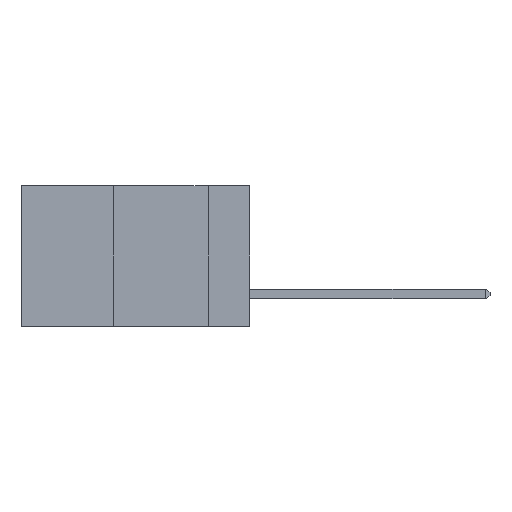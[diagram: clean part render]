
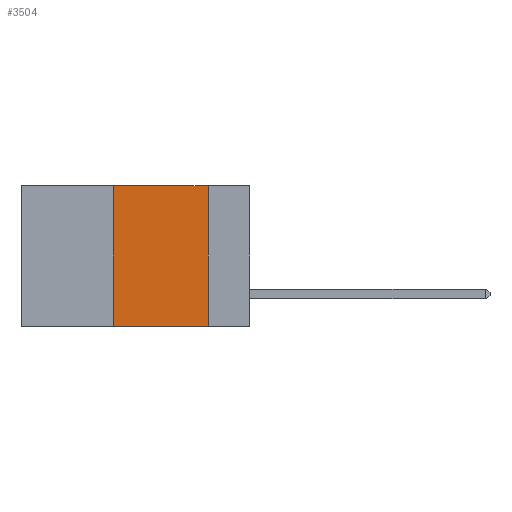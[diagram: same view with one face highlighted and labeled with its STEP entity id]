
A CAD part, left-side view. The second image highlights one B-rep face of the part: STEP entity #3504.
In plain terms, the highlighted planar face has unit normal (-1, 0, 0).
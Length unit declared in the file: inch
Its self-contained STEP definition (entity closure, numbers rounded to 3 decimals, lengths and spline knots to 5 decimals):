
#342 = CARTESIAN_POINT ( 'NONE',  ( 0., 0.36, 0. ) ) ;
#497 = CARTESIAN_POINT ( 'NONE',  ( 0., 0.36, 0. ) ) ;
#803 = VECTOR ( 'NONE', #12016, 39.37008 ) ;
#1072 = VECTOR ( 'NONE', #10085, 39.37008 ) ;
#1084 = CARTESIAN_POINT ( 'NONE',  ( 0., 0.6, 0. ) ) ;
#1309 = ORIENTED_EDGE ( 'NONE', *, *, #10374, .F. ) ;
#1501 = EDGE_CURVE ( 'NONE', #2262, #16297, #12782, .T. ) ;
#1684 = VECTOR ( 'NONE', #11362, 39.37008 ) ;
#2262 = VERTEX_POINT ( 'NONE', #497 ) ;
#2294 = DIRECTION ( 'NONE',  ( 1., 0., 0. ) ) ;
#2800 = CARTESIAN_POINT ( 'NONE',  ( 0., 0.11, -0.37 ) ) ;
#3504 = ADVANCED_FACE ( 'NONE', ( #16617 ), #7457, .F. ) ;
#3538 = ORIENTED_EDGE ( 'NONE', *, *, #1501, .F. ) ;
#4614 = LINE ( 'NONE', #10428, #803 ) ;
#4886 = LINE ( 'NONE', #7231, #1072 ) ;
#5921 = EDGE_CURVE ( 'NONE', #16297, #16323, #4614, .T. ) ;
#7231 = CARTESIAN_POINT ( 'NONE',  ( 0., 0.6, -0.37 ) ) ;
#7457 = PLANE ( 'NONE',  #16899 ) ;
#7774 = EDGE_LOOP ( 'NONE', ( #16067, #3538, #1309, #8228 ) ) ;
#8228 = ORIENTED_EDGE ( 'NONE', *, *, #13340, .T. ) ;
#8870 = DIRECTION ( 'NONE',  ( 0., 0., 1. ) ) ;
#9849 = CARTESIAN_POINT ( 'NONE',  ( 0., 0.11, 0. ) ) ;
#10085 = DIRECTION ( 'NONE',  ( 0., -1., 0. ) ) ;
#10374 = EDGE_CURVE ( 'NONE', #11148, #2262, #12689, .T. ) ;
#10428 = CARTESIAN_POINT ( 'NONE',  ( 0., 0.11, 0. ) ) ;
#11148 = VERTEX_POINT ( 'NONE', #15382 ) ;
#11362 = DIRECTION ( 'NONE',  ( 0., -1., 0. ) ) ;
#12016 = DIRECTION ( 'NONE',  ( 0., 0., -1. ) ) ;
#12689 = LINE ( 'NONE', #342, #15600 ) ;
#12782 = LINE ( 'NONE', #1084, #1684 ) ;
#12835 = DIRECTION ( 'NONE',  ( 0., 0., -1. ) ) ;
#13340 = EDGE_CURVE ( 'NONE', #11148, #16323, #4886, .T. ) ;
#15382 = CARTESIAN_POINT ( 'NONE',  ( 0., 0.36, -0.37 ) ) ;
#15600 = VECTOR ( 'NONE', #8870, 39.37008 ) ;
#16067 = ORIENTED_EDGE ( 'NONE', *, *, #5921, .F. ) ;
#16297 = VERTEX_POINT ( 'NONE', #9849 ) ;
#16323 = VERTEX_POINT ( 'NONE', #2800 ) ;
#16412 = CARTESIAN_POINT ( 'NONE',  ( 0., 0.6, 0. ) ) ;
#16617 = FACE_OUTER_BOUND ( 'NONE', #7774, .T. ) ;
#16899 = AXIS2_PLACEMENT_3D ( 'NONE', #16412, #2294, #12835 ) ;
